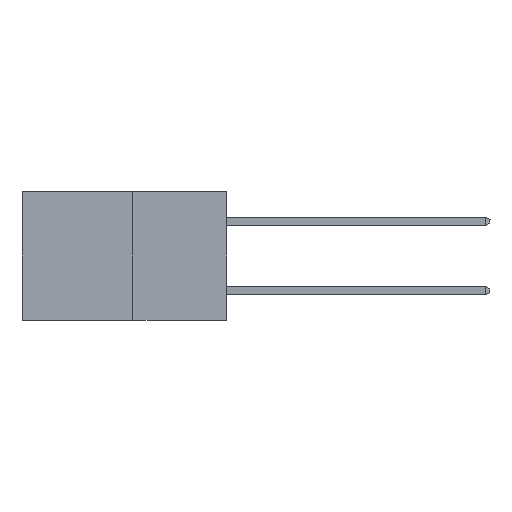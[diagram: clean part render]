
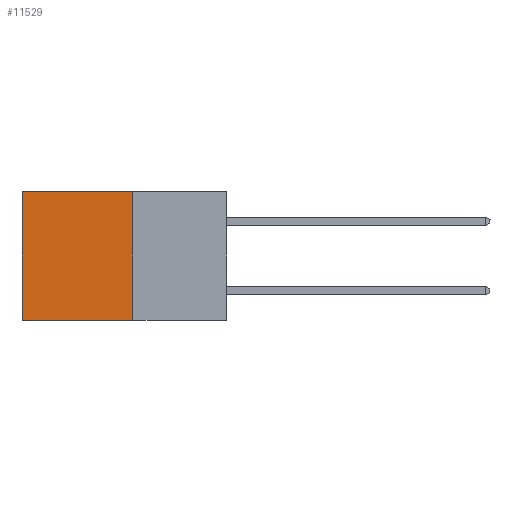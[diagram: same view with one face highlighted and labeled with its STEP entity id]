
A CAD part, left-side view. The second image highlights one B-rep face of the part: STEP entity #11529.
In plain terms, the highlighted planar face has unit normal (-1, 0, 0).
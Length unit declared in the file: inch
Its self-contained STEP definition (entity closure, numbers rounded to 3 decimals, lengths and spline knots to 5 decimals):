
#376 = PLANE ( 'NONE',  #1187 ) ;
#830 = ORIENTED_EDGE ( 'NONE', *, *, #12006, .T. ) ;
#905 = VERTEX_POINT ( 'NONE', #3452 ) ;
#1187 = AXIS2_PLACEMENT_3D ( 'NONE', #4359, #7246, #1366 ) ;
#1366 = DIRECTION ( 'NONE',  ( 0., 0., -1. ) ) ;
#1556 = CARTESIAN_POINT ( 'NONE',  ( 0.277, 0.27, -0.37 ) ) ;
#1654 = LINE ( 'NONE', #1556, #4331 ) ;
#2012 = VERTEX_POINT ( 'NONE', #5408 ) ;
#2722 = ORIENTED_EDGE ( 'NONE', *, *, #8744, .F. ) ;
#2846 = ORIENTED_EDGE ( 'NONE', *, *, #5152, .F. ) ;
#3244 = VERTEX_POINT ( 'NONE', #8427 ) ;
#3411 = VERTEX_POINT ( 'NONE', #10242 ) ;
#3452 = CARTESIAN_POINT ( 'NONE',  ( 0.277, 0.27, -0.37 ) ) ;
#3994 = DIRECTION ( 'NONE',  ( 0., 0., -1. ) ) ;
#4331 = VECTOR ( 'NONE', #9372, 39.37008 ) ;
#4359 = CARTESIAN_POINT ( 'NONE',  ( 0.277, 0.27, -0.37 ) ) ;
#5152 = EDGE_CURVE ( 'NONE', #3411, #905, #11862, .T. ) ;
#5408 = CARTESIAN_POINT ( 'NONE',  ( 0.277, 0.59, -0.37 ) ) ;
#6007 = DIRECTION ( 'NONE',  ( 0., 0., -1. ) ) ;
#6267 = CARTESIAN_POINT ( 'NONE',  ( 0.277, 0.27, -0.37 ) ) ;
#6750 = VECTOR ( 'NONE', #6007, 39.37008 ) ;
#7246 = DIRECTION ( 'NONE',  ( 1., 0., 0. ) ) ;
#7908 = CARTESIAN_POINT ( 'NONE',  ( 0.277, 0.59, -0.37 ) ) ;
#8245 = ORIENTED_EDGE ( 'NONE', *, *, #12335, .T. ) ;
#8382 = DIRECTION ( 'NONE',  ( 0., 1., 0. ) ) ;
#8427 = CARTESIAN_POINT ( 'NONE',  ( 0.277, 0.59, 0. ) ) ;
#8474 = VECTOR ( 'NONE', #3994, 39.37008 ) ;
#8744 = EDGE_CURVE ( 'NONE', #905, #2012, #1654, .T. ) ;
#8899 = FACE_OUTER_BOUND ( 'NONE', #10704, .T. ) ;
#9372 = DIRECTION ( 'NONE',  ( 0., 1., 0. ) ) ;
#9973 = LINE ( 'NONE', #12211, #12188 ) ;
#10242 = CARTESIAN_POINT ( 'NONE',  ( 0.277, 0.27, 0. ) ) ;
#10704 = EDGE_LOOP ( 'NONE', ( #830, #2722, #2846, #8245 ) ) ;
#11337 = LINE ( 'NONE', #7908, #8474 ) ;
#11529 = ADVANCED_FACE ( 'NONE', ( #8899 ), #376, .F. ) ;
#11862 = LINE ( 'NONE', #6267, #6750 ) ;
#12006 = EDGE_CURVE ( 'NONE', #3244, #2012, #11337, .T. ) ;
#12188 = VECTOR ( 'NONE', #8382, 39.37008 ) ;
#12211 = CARTESIAN_POINT ( 'NONE',  ( 0.277, 0.27, 0. ) ) ;
#12335 = EDGE_CURVE ( 'NONE', #3411, #3244, #9973, .T. ) ;
